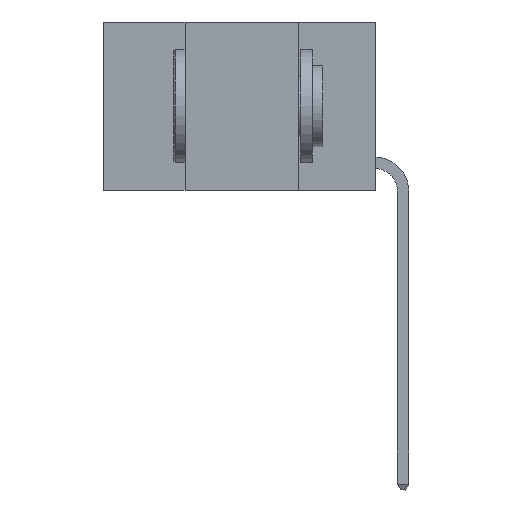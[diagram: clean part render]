
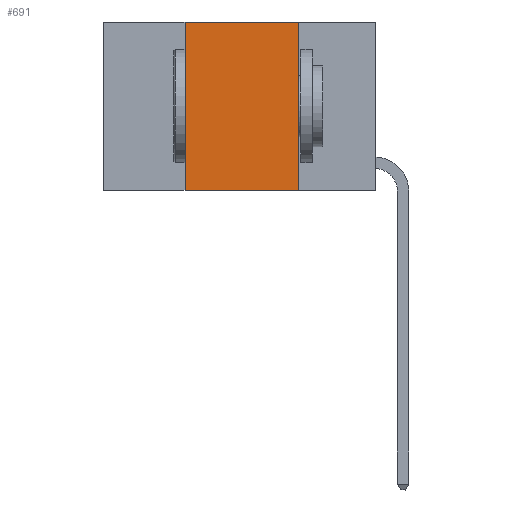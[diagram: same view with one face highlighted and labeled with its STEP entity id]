
A CAD part, left-side view. The second image highlights one B-rep face of the part: STEP entity #691.
In plain terms, the highlighted planar face has unit normal (-1, 0, 0).
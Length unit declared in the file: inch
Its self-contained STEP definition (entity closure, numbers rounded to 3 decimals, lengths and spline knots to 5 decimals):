
#65 = DIRECTION ( 'NONE',  ( 1., 0., 0. ) ) ;
#323 = ORIENTED_EDGE ( 'NONE', *, *, #8273, .F. ) ;
#691 = ADVANCED_FACE ( 'NONE', ( #12580 ), #7205, .F. ) ;
#1360 = CARTESIAN_POINT ( 'NONE',  ( 0., 0.17, 0. ) ) ;
#1890 = CARTESIAN_POINT ( 'NONE',  ( 0., 0.6, 0. ) ) ;
#2095 = LINE ( 'NONE', #9668, #13288 ) ;
#2126 = CARTESIAN_POINT ( 'NONE',  ( 0., 0.42, -0.37 ) ) ;
#2707 = VERTEX_POINT ( 'NONE', #2126 ) ;
#3316 = CARTESIAN_POINT ( 'NONE',  ( 0., 0.6, 0. ) ) ;
#3444 = VERTEX_POINT ( 'NONE', #9597 ) ;
#3475 = ORIENTED_EDGE ( 'NONE', *, *, #9198, .T. ) ;
#4110 = DIRECTION ( 'NONE',  ( 0., -1., 0. ) ) ;
#4117 = LINE ( 'NONE', #1360, #12045 ) ;
#4147 = CARTESIAN_POINT ( 'NONE',  ( 0., 0.42, 0. ) ) ;
#4791 = AXIS2_PLACEMENT_3D ( 'NONE', #3316, #65, #6745 ) ;
#5069 = VECTOR ( 'NONE', #4110, 39.37008 ) ;
#5086 = EDGE_CURVE ( 'NONE', #12271, #8279, #7852, .T. ) ;
#5269 = DIRECTION ( 'NONE',  ( 0., 0., 1. ) ) ;
#6012 = ORIENTED_EDGE ( 'NONE', *, *, #11626, .F. ) ;
#6309 = CARTESIAN_POINT ( 'NONE',  ( 0., 0.17, 0. ) ) ;
#6745 = DIRECTION ( 'NONE',  ( 0., 0., -1. ) ) ;
#7188 = LINE ( 'NONE', #4147, #9701 ) ;
#7205 = PLANE ( 'NONE',  #4791 ) ;
#7852 = LINE ( 'NONE', #1890, #5069 ) ;
#8273 = EDGE_CURVE ( 'NONE', #2707, #12271, #7188, .T. ) ;
#8279 = VERTEX_POINT ( 'NONE', #6309 ) ;
#8612 = DIRECTION ( 'NONE',  ( 0., -1., 0. ) ) ;
#9198 = EDGE_CURVE ( 'NONE', #2707, #3444, #2095, .T. ) ;
#9597 = CARTESIAN_POINT ( 'NONE',  ( 0., 0.17, -0.37 ) ) ;
#9668 = CARTESIAN_POINT ( 'NONE',  ( 0., 0.6, -0.37 ) ) ;
#9701 = VECTOR ( 'NONE', #5269, 39.37008 ) ;
#10049 = DIRECTION ( 'NONE',  ( 0., 0., -1. ) ) ;
#11399 = CARTESIAN_POINT ( 'NONE',  ( 0., 0.42, 0. ) ) ;
#11626 = EDGE_CURVE ( 'NONE', #8279, #3444, #4117, .T. ) ;
#11755 = ORIENTED_EDGE ( 'NONE', *, *, #5086, .F. ) ;
#12045 = VECTOR ( 'NONE', #10049, 39.37008 ) ;
#12271 = VERTEX_POINT ( 'NONE', #11399 ) ;
#12580 = FACE_OUTER_BOUND ( 'NONE', #12748, .T. ) ;
#12748 = EDGE_LOOP ( 'NONE', ( #6012, #11755, #323, #3475 ) ) ;
#13288 = VECTOR ( 'NONE', #8612, 39.37008 ) ;
